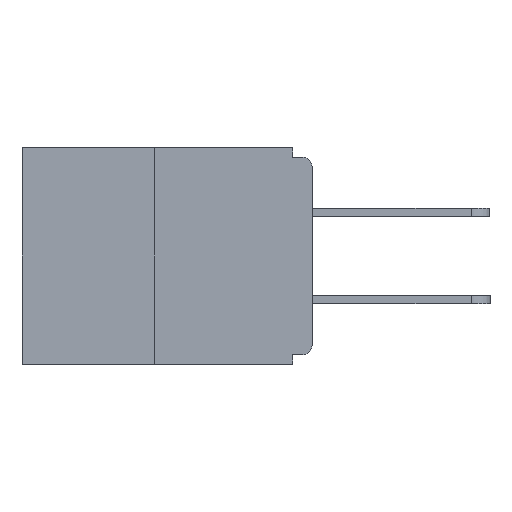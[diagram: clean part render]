
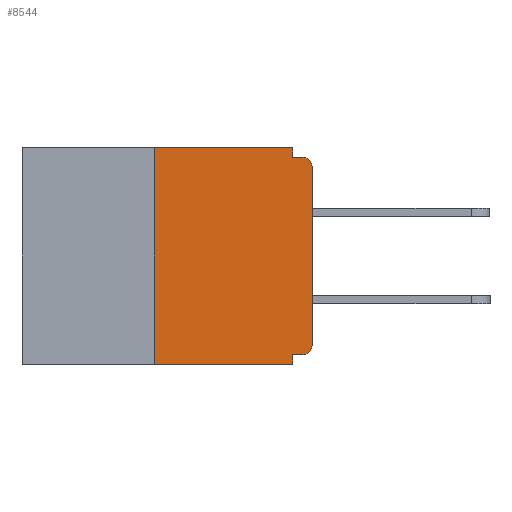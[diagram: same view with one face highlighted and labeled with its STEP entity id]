
A CAD part, left-side view. The second image highlights one B-rep face of the part: STEP entity #8544.
In plain terms, the highlighted planar face has unit normal (-1, 0, 0).
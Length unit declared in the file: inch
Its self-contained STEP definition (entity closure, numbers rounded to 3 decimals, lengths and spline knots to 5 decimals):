
#25 = DIRECTION ( 'NONE',  ( 1., 0., 0. ) ) ;
#62 = CARTESIAN_POINT ( 'NONE',  ( 0., 0.015, -0.03 ) ) ;
#86 = EDGE_CURVE ( 'NONE', #5117, #561, #2280, .T. ) ;
#159 = LINE ( 'NONE', #9405, #10253 ) ;
#250 = EDGE_CURVE ( 'NONE', #5335, #2001, #4889, .T. ) ;
#523 = ORIENTED_EDGE ( 'NONE', *, *, #1660, .F. ) ;
#561 = VERTEX_POINT ( 'NONE', #4518 ) ;
#1116 = VECTOR ( 'NONE', #5310, 39.37008 ) ;
#1154 = LINE ( 'NONE', #1833, #1116 ) ;
#1233 = CARTESIAN_POINT ( 'NONE',  ( 0., 0.015, -0.328 ) ) ;
#1409 = VERTEX_POINT ( 'NONE', #10699 ) ;
#1535 = CARTESIAN_POINT ( 'NONE',  ( 0., 0.25, 0. ) ) ;
#1660 = EDGE_CURVE ( 'NONE', #2285, #5655, #5505, .T. ) ;
#1736 = DIRECTION ( 'NONE',  ( 0., -1., 0. ) ) ;
#1833 = CARTESIAN_POINT ( 'NONE',  ( 0., 0., 0. ) ) ;
#1840 = DIRECTION ( 'NONE',  ( 0., -1., 0. ) ) ;
#1927 = FACE_OUTER_BOUND ( 'NONE', #9418, .T. ) ;
#1963 = CIRCLE ( 'NONE', #4874, 0.015 ) ;
#2001 = VERTEX_POINT ( 'NONE', #7486 ) ;
#2158 = ORIENTED_EDGE ( 'NONE', *, *, #86, .F. ) ;
#2280 = LINE ( 'NONE', #1535, #10602 ) ;
#2285 = VERTEX_POINT ( 'NONE', #7829 ) ;
#2570 = CARTESIAN_POINT ( 'NONE',  ( 0., 0.031, -0.343 ) ) ;
#2661 = ORIENTED_EDGE ( 'NONE', *, *, #250, .T. ) ;
#2812 = CARTESIAN_POINT ( 'NONE',  ( 0., 0.46, -0.343 ) ) ;
#2911 = ORIENTED_EDGE ( 'NONE', *, *, #6182, .T. ) ;
#3070 = VERTEX_POINT ( 'NONE', #8035 ) ;
#3175 = CARTESIAN_POINT ( 'NONE',  ( 0., 0.015, -0.313 ) ) ;
#3282 = CARTESIAN_POINT ( 'NONE',  ( 0., 0.46, 0. ) ) ;
#3395 = CARTESIAN_POINT ( 'NONE',  ( 0., 0., -0.03 ) ) ;
#3515 = LINE ( 'NONE', #2812, #4180 ) ;
#3885 = DIRECTION ( 'NONE',  ( 0., 0., -1. ) ) ;
#4180 = VECTOR ( 'NONE', #1736, 39.37008 ) ;
#4296 = EDGE_CURVE ( 'NONE', #561, #4417, #7519, .T. ) ;
#4354 = VECTOR ( 'NONE', #6715, 39.37008 ) ;
#4417 = VERTEX_POINT ( 'NONE', #5315 ) ;
#4518 = CARTESIAN_POINT ( 'NONE',  ( 0., 0.25, 0. ) ) ;
#4874 = AXIS2_PLACEMENT_3D ( 'NONE', #3175, #5658, #4936 ) ;
#4889 = CIRCLE ( 'NONE', #5777, 0.015 ) ;
#4904 = CARTESIAN_POINT ( 'NONE',  ( 0., 0.031, 0. ) ) ;
#4936 = DIRECTION ( 'NONE',  ( 0., 0., -1. ) ) ;
#5102 = DIRECTION ( 'NONE',  ( 0., 0., 1. ) ) ;
#5117 = VERTEX_POINT ( 'NONE', #5547 ) ;
#5177 = EDGE_CURVE ( 'NONE', #7376, #3070, #1963, .T. ) ;
#5310 = DIRECTION ( 'NONE',  ( 0., 0., 1. ) ) ;
#5315 = CARTESIAN_POINT ( 'NONE',  ( 0., 0.031, 0. ) ) ;
#5335 = VERTEX_POINT ( 'NONE', #3395 ) ;
#5505 = LINE ( 'NONE', #9924, #8260 ) ;
#5547 = CARTESIAN_POINT ( 'NONE',  ( 0., 0.25, -0.343 ) ) ;
#5655 = VERTEX_POINT ( 'NONE', #2570 ) ;
#5658 = DIRECTION ( 'NONE',  ( -1., 0., 0. ) ) ;
#5759 = ORIENTED_EDGE ( 'NONE', *, *, #6867, .F. ) ;
#5777 = AXIS2_PLACEMENT_3D ( 'NONE', #62, #9726, #10665 ) ;
#5845 = CARTESIAN_POINT ( 'NONE',  ( 0., 0., -0.328 ) ) ;
#6182 = EDGE_CURVE ( 'NONE', #5117, #5655, #3515, .T. ) ;
#6281 = ORIENTED_EDGE ( 'NONE', *, *, #5177, .T. ) ;
#6392 = EDGE_CURVE ( 'NONE', #7376, #2285, #11193, .T. ) ;
#6460 = LINE ( 'NONE', #4904, #7377 ) ;
#6715 = DIRECTION ( 'NONE',  ( 0., 1., 0. ) ) ;
#6867 = EDGE_CURVE ( 'NONE', #1409, #2001, #159, .T. ) ;
#7005 = ORIENTED_EDGE ( 'NONE', *, *, #9991, .T. ) ;
#7154 = AXIS2_PLACEMENT_3D ( 'NONE', #9576, #25, #10688 ) ;
#7376 = VERTEX_POINT ( 'NONE', #1233 ) ;
#7377 = VECTOR ( 'NONE', #3885, 39.37008 ) ;
#7486 = CARTESIAN_POINT ( 'NONE',  ( 0., 0.015, -0.015 ) ) ;
#7519 = LINE ( 'NONE', #3282, #8741 ) ;
#7655 = EDGE_CURVE ( 'NONE', #4417, #1409, #6460, .T. ) ;
#7829 = CARTESIAN_POINT ( 'NONE',  ( 0., 0.031, -0.328 ) ) ;
#8035 = CARTESIAN_POINT ( 'NONE',  ( 0., 0., -0.313 ) ) ;
#8048 = DIRECTION ( 'NONE',  ( 0., 0., -1. ) ) ;
#8181 = ORIENTED_EDGE ( 'NONE', *, *, #7655, .F. ) ;
#8260 = VECTOR ( 'NONE', #8048, 39.37008 ) ;
#8544 = ADVANCED_FACE ( 'NONE', ( #1927 ), #9807, .F. ) ;
#8741 = VECTOR ( 'NONE', #9310, 39.37008 ) ;
#9310 = DIRECTION ( 'NONE',  ( 0., -1., 0. ) ) ;
#9405 = CARTESIAN_POINT ( 'NONE',  ( 0., 0., -0.015 ) ) ;
#9418 = EDGE_LOOP ( 'NONE', ( #10745, #2158, #2911, #523, #9993, #6281, #7005, #2661, #5759, #8181 ) ) ;
#9576 = CARTESIAN_POINT ( 'NONE',  ( 0., 0.46, 0. ) ) ;
#9726 = DIRECTION ( 'NONE',  ( -1., 0., 0. ) ) ;
#9807 = PLANE ( 'NONE',  #7154 ) ;
#9924 = CARTESIAN_POINT ( 'NONE',  ( 0., 0.031, -0.343 ) ) ;
#9991 = EDGE_CURVE ( 'NONE', #3070, #5335, #1154, .T. ) ;
#9993 = ORIENTED_EDGE ( 'NONE', *, *, #6392, .F. ) ;
#10253 = VECTOR ( 'NONE', #1840, 39.37008 ) ;
#10602 = VECTOR ( 'NONE', #5102, 39.37008 ) ;
#10665 = DIRECTION ( 'NONE',  ( 0., 0., -1. ) ) ;
#10688 = DIRECTION ( 'NONE',  ( 0., 0., -1. ) ) ;
#10699 = CARTESIAN_POINT ( 'NONE',  ( 0., 0.031, -0.015 ) ) ;
#10745 = ORIENTED_EDGE ( 'NONE', *, *, #4296, .F. ) ;
#11193 = LINE ( 'NONE', #5845, #4354 ) ;
